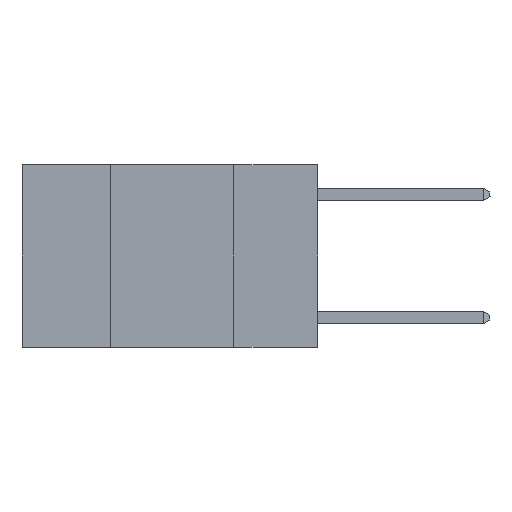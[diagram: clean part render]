
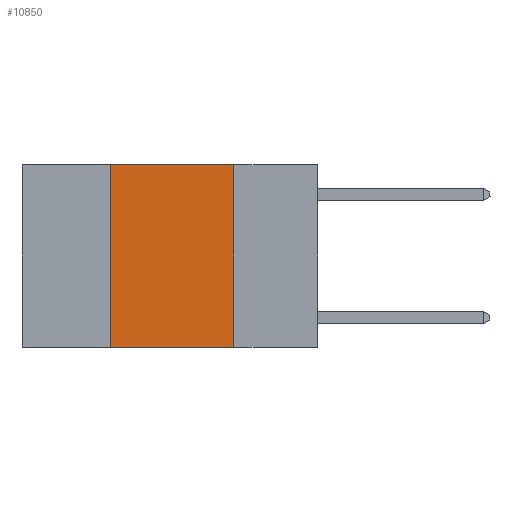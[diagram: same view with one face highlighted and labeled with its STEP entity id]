
A CAD part, left-side view. The second image highlights one B-rep face of the part: STEP entity #10850.
In plain terms, the highlighted planar face has unit normal (-1, 0, 0).
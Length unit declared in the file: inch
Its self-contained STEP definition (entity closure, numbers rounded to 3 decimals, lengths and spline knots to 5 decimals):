
#282 = VECTOR ( 'NONE', #2273, 39.37008 ) ;
#296 = CARTESIAN_POINT ( 'NONE',  ( 0., 0.6, -0.37 ) ) ;
#958 = LINE ( 'NONE', #6900, #282 ) ;
#1213 = LINE ( 'NONE', #3555, #15024 ) ;
#1684 = EDGE_CURVE ( 'NONE', #4404, #14634, #1213, .T. ) ;
#1860 = DIRECTION ( 'NONE',  ( 0., 0., -1. ) ) ;
#2273 = DIRECTION ( 'NONE',  ( 0., 0., 1. ) ) ;
#2838 = CARTESIAN_POINT ( 'NONE',  ( 0., 0.17, -0.37 ) ) ;
#3555 = CARTESIAN_POINT ( 'NONE',  ( 0., 0.17, 0. ) ) ;
#3678 = CARTESIAN_POINT ( 'NONE',  ( 0., 0.42, -0.37 ) ) ;
#3778 = EDGE_CURVE ( 'NONE', #12125, #9773, #958, .T. ) ;
#3941 = DIRECTION ( 'NONE',  ( 0., -1., 0. ) ) ;
#4398 = AXIS2_PLACEMENT_3D ( 'NONE', #7399, #14353, #1860 ) ;
#4404 = VERTEX_POINT ( 'NONE', #8912 ) ;
#4537 = DIRECTION ( 'NONE',  ( 0., -1., 0. ) ) ;
#5468 = ORIENTED_EDGE ( 'NONE', *, *, #13922, .T. ) ;
#5471 = ORIENTED_EDGE ( 'NONE', *, *, #1684, .F. ) ;
#5490 = EDGE_LOOP ( 'NONE', ( #5471, #12866, #13971, #5468 ) ) ;
#6115 = FACE_OUTER_BOUND ( 'NONE', #5490, .T. ) ;
#6900 = CARTESIAN_POINT ( 'NONE',  ( 0., 0.42, 0. ) ) ;
#7134 = EDGE_CURVE ( 'NONE', #9773, #4404, #12560, .T. ) ;
#7399 = CARTESIAN_POINT ( 'NONE',  ( 0., 0.6, 0. ) ) ;
#8214 = DIRECTION ( 'NONE',  ( 0., 0., -1. ) ) ;
#8912 = CARTESIAN_POINT ( 'NONE',  ( 0., 0.17, 0. ) ) ;
#9773 = VERTEX_POINT ( 'NONE', #11439 ) ;
#10850 = ADVANCED_FACE ( 'NONE', ( #6115 ), #12360, .F. ) ;
#10970 = VECTOR ( 'NONE', #4537, 39.37008 ) ;
#11439 = CARTESIAN_POINT ( 'NONE',  ( 0., 0.42, 0. ) ) ;
#11573 = CARTESIAN_POINT ( 'NONE',  ( 0., 0.6, 0. ) ) ;
#11816 = LINE ( 'NONE', #296, #13822 ) ;
#12125 = VERTEX_POINT ( 'NONE', #3678 ) ;
#12360 = PLANE ( 'NONE',  #4398 ) ;
#12560 = LINE ( 'NONE', #11573, #10970 ) ;
#12866 = ORIENTED_EDGE ( 'NONE', *, *, #7134, .F. ) ;
#13822 = VECTOR ( 'NONE', #3941, 39.37008 ) ;
#13922 = EDGE_CURVE ( 'NONE', #12125, #14634, #11816, .T. ) ;
#13971 = ORIENTED_EDGE ( 'NONE', *, *, #3778, .F. ) ;
#14353 = DIRECTION ( 'NONE',  ( 1., 0., 0. ) ) ;
#14634 = VERTEX_POINT ( 'NONE', #2838 ) ;
#15024 = VECTOR ( 'NONE', #8214, 39.37008 ) ;
